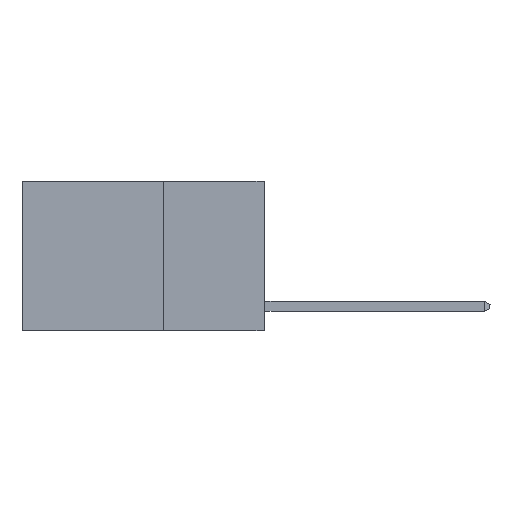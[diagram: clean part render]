
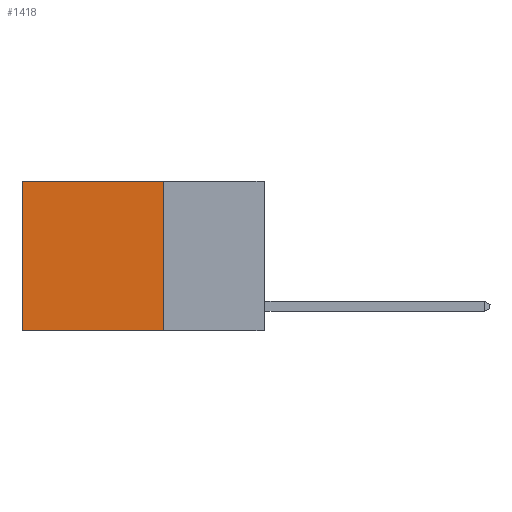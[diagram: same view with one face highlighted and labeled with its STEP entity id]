
A CAD part, left-side view. The second image highlights one B-rep face of the part: STEP entity #1418.
In plain terms, the highlighted planar face has unit normal (-1, 0, 0).
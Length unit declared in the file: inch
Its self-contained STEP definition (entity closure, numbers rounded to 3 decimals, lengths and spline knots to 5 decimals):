
#931 = ORIENTED_EDGE ( 'NONE', *, *, #26638, .F. ) ;
#1418 = ADVANCED_FACE ( 'NONE', ( #23642 ), #10636, .F. ) ;
#3038 = CARTESIAN_POINT ( 'NONE',  ( 0.2625, 0.6, 0. ) ) ;
#4076 = CARTESIAN_POINT ( 'NONE',  ( 0.2625, 0.25, 0. ) ) ;
#4353 = DIRECTION ( 'NONE',  ( 0., 1., 0. ) ) ;
#5164 = CARTESIAN_POINT ( 'NONE',  ( 0.2625, 0.25, -0.37 ) ) ;
#6027 = CARTESIAN_POINT ( 'NONE',  ( 0.2625, 0.6, 0. ) ) ;
#6122 = EDGE_CURVE ( 'NONE', #21086, #17661, #13439, .T. ) ;
#6447 = LINE ( 'NONE', #5164, #18156 ) ;
#6774 = ORIENTED_EDGE ( 'NONE', *, *, #6122, .T. ) ;
#7400 = DIRECTION ( 'NONE',  ( 0., 1., 0. ) ) ;
#7569 = VECTOR ( 'NONE', #28028, 39.37008 ) ;
#7970 = AXIS2_PLACEMENT_3D ( 'NONE', #4076, #8514, #23926 ) ;
#8514 = DIRECTION ( 'NONE',  ( 1., 0., 0. ) ) ;
#8698 = CARTESIAN_POINT ( 'NONE',  ( 0.2625, 0.25, 0. ) ) ;
#8943 = EDGE_LOOP ( 'NONE', ( #6774, #931, #10552, #14013 ) ) ;
#9861 = CARTESIAN_POINT ( 'NONE',  ( 0.2625, 0.25, 0. ) ) ;
#10047 = LINE ( 'NONE', #8698, #20370 ) ;
#10552 = ORIENTED_EDGE ( 'NONE', *, *, #25606, .F. ) ;
#10636 = PLANE ( 'NONE',  #7970 ) ;
#11853 = CARTESIAN_POINT ( 'NONE',  ( 0.2625, 0.25, -0.37 ) ) ;
#12082 = DIRECTION ( 'NONE',  ( 0., 0., -1. ) ) ;
#13439 = LINE ( 'NONE', #6027, #7569 ) ;
#14013 = ORIENTED_EDGE ( 'NONE', *, *, #23206, .T. ) ;
#17655 = CARTESIAN_POINT ( 'NONE',  ( 0.2625, 0.25, 0. ) ) ;
#17661 = VERTEX_POINT ( 'NONE', #18374 ) ;
#18156 = VECTOR ( 'NONE', #7400, 39.37008 ) ;
#18374 = CARTESIAN_POINT ( 'NONE',  ( 0.2625, 0.6, -0.37 ) ) ;
#18571 = VECTOR ( 'NONE', #12082, 39.37008 ) ;
#18798 = VERTEX_POINT ( 'NONE', #17655 ) ;
#19256 = LINE ( 'NONE', #9861, #18571 ) ;
#20370 = VECTOR ( 'NONE', #4353, 39.37008 ) ;
#20476 = VERTEX_POINT ( 'NONE', #11853 ) ;
#21086 = VERTEX_POINT ( 'NONE', #3038 ) ;
#23206 = EDGE_CURVE ( 'NONE', #18798, #21086, #10047, .T. ) ;
#23642 = FACE_OUTER_BOUND ( 'NONE', #8943, .T. ) ;
#23926 = DIRECTION ( 'NONE',  ( 0., 0., -1. ) ) ;
#25606 = EDGE_CURVE ( 'NONE', #18798, #20476, #19256, .T. ) ;
#26638 = EDGE_CURVE ( 'NONE', #20476, #17661, #6447, .T. ) ;
#28028 = DIRECTION ( 'NONE',  ( 0., 0., -1. ) ) ;
